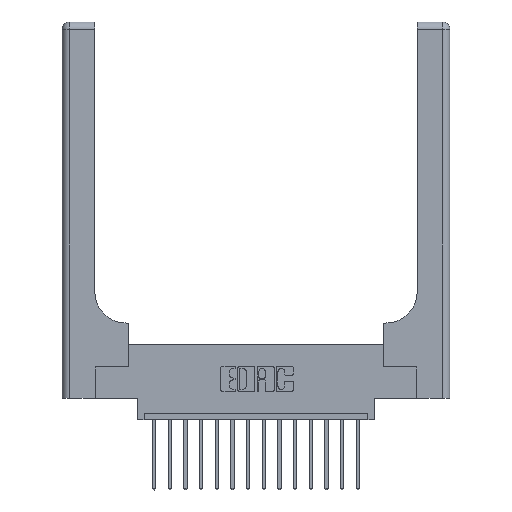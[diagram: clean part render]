
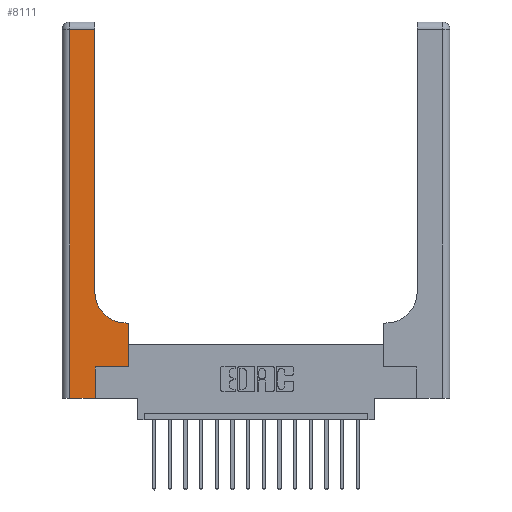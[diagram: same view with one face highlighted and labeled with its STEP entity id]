
A CAD part, top view. The second image highlights one B-rep face of the part: STEP entity #8111.
In plain terms, the highlighted planar face has unit normal (0, 0, 1).
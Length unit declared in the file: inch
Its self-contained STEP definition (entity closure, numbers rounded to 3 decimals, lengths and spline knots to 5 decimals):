
#152 = CARTESIAN_POINT ( 'NONE',  ( 0.528, 0.25, 0.37 ) ) ;
#192 = DIRECTION ( 'NONE',  ( -1., 0., 0. ) ) ;
#305 = CARTESIAN_POINT ( 'NONE',  ( 0.26, 0.6, 0.37 ) ) ;
#366 = LINE ( 'NONE', #9118, #2291 ) ;
#471 = VECTOR ( 'NONE', #9569, 39.37008 ) ;
#766 = DIRECTION ( 'NONE',  ( 0., 0., -1. ) ) ;
#920 = VECTOR ( 'NONE', #2938, 39.37008 ) ;
#1164 = CARTESIAN_POINT ( 'NONE',  ( 0.06, 2.94, 0.37 ) ) ;
#1316 = EDGE_CURVE ( 'NONE', #1974, #9675, #3319, .T. ) ;
#1322 = CARTESIAN_POINT ( 'NONE',  ( 0.265, 0.25, 0.37 ) ) ;
#1799 = ORIENTED_EDGE ( 'NONE', *, *, #17254, .T. ) ;
#1974 = VERTEX_POINT ( 'NONE', #4221 ) ;
#1991 = LINE ( 'NONE', #2902, #6267 ) ;
#2071 = ORIENTED_EDGE ( 'NONE', *, *, #2751, .T. ) ;
#2113 = VERTEX_POINT ( 'NONE', #3090 ) ;
#2291 = VECTOR ( 'NONE', #10376, 39.37008 ) ;
#2452 = VECTOR ( 'NONE', #16684, 39.37008 ) ;
#2751 = EDGE_CURVE ( 'NONE', #2113, #12138, #12316, .T. ) ;
#2767 = DIRECTION ( 'NONE',  ( -1., 0., 0. ) ) ;
#2902 = CARTESIAN_POINT ( 'NONE',  ( 0., 0., 0.37 ) ) ;
#2938 = DIRECTION ( 'NONE',  ( 0., 1., 0. ) ) ;
#3090 = CARTESIAN_POINT ( 'NONE',  ( 0.51, 0.6, 0.37 ) ) ;
#3319 = LINE ( 'NONE', #8076, #12979 ) ;
#3338 = LINE ( 'NONE', #7397, #4818 ) ;
#3785 = CARTESIAN_POINT ( 'NONE',  ( 0.06, 0., 0.37 ) ) ;
#4067 = CARTESIAN_POINT ( 'NONE',  ( 0.26, 0.85, 0.37 ) ) ;
#4221 = CARTESIAN_POINT ( 'NONE',  ( 0.26, 2.94, 0.37 ) ) ;
#4362 = AXIS2_PLACEMENT_3D ( 'NONE', #6169, #766, #14576 ) ;
#4409 = AXIS2_PLACEMENT_3D ( 'NONE', #4987, #9098, #10469 ) ;
#4413 = CARTESIAN_POINT ( 'NONE',  ( 0.265, 0., 0.37 ) ) ;
#4563 = ORIENTED_EDGE ( 'NONE', *, *, #13042, .T. ) ;
#4818 = VECTOR ( 'NONE', #16967, 39.37008 ) ;
#4987 = CARTESIAN_POINT ( 'NONE',  ( 0.51, 0.85, 0.37 ) ) ;
#5418 = VECTOR ( 'NONE', #192, 39.37008 ) ;
#5657 = LINE ( 'NONE', #8404, #2452 ) ;
#5658 = FACE_OUTER_BOUND ( 'NONE', #10429, .T. ) ;
#6169 = CARTESIAN_POINT ( 'NONE',  ( 0., 3., 0.37 ) ) ;
#6267 = VECTOR ( 'NONE', #12324, 39.37008 ) ;
#6347 = ORIENTED_EDGE ( 'NONE', *, *, #8792, .T. ) ;
#6517 = ORIENTED_EDGE ( 'NONE', *, *, #11874, .T. ) ;
#7108 = CARTESIAN_POINT ( 'NONE',  ( 0.528, 0.25, 0.37 ) ) ;
#7116 = ORIENTED_EDGE ( 'NONE', *, *, #14602, .T. ) ;
#7306 = LINE ( 'NONE', #16397, #471 ) ;
#7397 = CARTESIAN_POINT ( 'NONE',  ( 0.265, 0.25, 0.37 ) ) ;
#7501 = VERTEX_POINT ( 'NONE', #152 ) ;
#8076 = CARTESIAN_POINT ( 'NONE',  ( 0., 2.94, 0.37 ) ) ;
#8111 = ADVANCED_FACE ( 'NONE', ( #5658 ), #16853, .F. ) ;
#8186 = ORIENTED_EDGE ( 'NONE', *, *, #16167, .T. ) ;
#8404 = CARTESIAN_POINT ( 'NONE',  ( 0.265, 0., 0.37 ) ) ;
#8792 = EDGE_CURVE ( 'NONE', #13490, #2113, #15942, .T. ) ;
#9098 = DIRECTION ( 'NONE',  ( 0., 0., -1. ) ) ;
#9118 = CARTESIAN_POINT ( 'NONE',  ( 0.26, 3., 0.37 ) ) ;
#9569 = DIRECTION ( 'NONE',  ( 0., -1., 0. ) ) ;
#9675 = VERTEX_POINT ( 'NONE', #1164 ) ;
#9865 = VERTEX_POINT ( 'NONE', #4413 ) ;
#10376 = DIRECTION ( 'NONE',  ( 0., 1., 0. ) ) ;
#10429 = EDGE_LOOP ( 'NONE', ( #6517, #15069, #8186, #7116, #10911, #4563, #1799, #6347, #2071 ) ) ;
#10469 = DIRECTION ( 'NONE',  ( 1., 0., 0. ) ) ;
#10911 = ORIENTED_EDGE ( 'NONE', *, *, #13652, .T. ) ;
#11874 = EDGE_CURVE ( 'NONE', #12138, #1974, #366, .T. ) ;
#12075 = CARTESIAN_POINT ( 'NONE',  ( 0.528, 0.6, 0.37 ) ) ;
#12138 = VERTEX_POINT ( 'NONE', #4067 ) ;
#12316 = CIRCLE ( 'NONE', #4409, 0.25 ) ;
#12324 = DIRECTION ( 'NONE',  ( 1., 0., 0. ) ) ;
#12979 = VECTOR ( 'NONE', #2767, 39.37008 ) ;
#13042 = EDGE_CURVE ( 'NONE', #17595, #7501, #3338, .T. ) ;
#13490 = VERTEX_POINT ( 'NONE', #12075 ) ;
#13652 = EDGE_CURVE ( 'NONE', #9865, #17595, #5657, .T. ) ;
#13932 = VERTEX_POINT ( 'NONE', #3785 ) ;
#14576 = DIRECTION ( 'NONE',  ( -1., 0., 0. ) ) ;
#14602 = EDGE_CURVE ( 'NONE', #13932, #9865, #1991, .T. ) ;
#15069 = ORIENTED_EDGE ( 'NONE', *, *, #1316, .T. ) ;
#15942 = LINE ( 'NONE', #305, #5418 ) ;
#16167 = EDGE_CURVE ( 'NONE', #9675, #13932, #7306, .T. ) ;
#16397 = CARTESIAN_POINT ( 'NONE',  ( 0.06, 3., 0.37 ) ) ;
#16684 = DIRECTION ( 'NONE',  ( 0., 1., 0. ) ) ;
#16853 = PLANE ( 'NONE',  #4362 ) ;
#16967 = DIRECTION ( 'NONE',  ( 1., 0., 0. ) ) ;
#17254 = EDGE_CURVE ( 'NONE', #7501, #13490, #17472, .T. ) ;
#17472 = LINE ( 'NONE', #7108, #920 ) ;
#17595 = VERTEX_POINT ( 'NONE', #1322 ) ;
